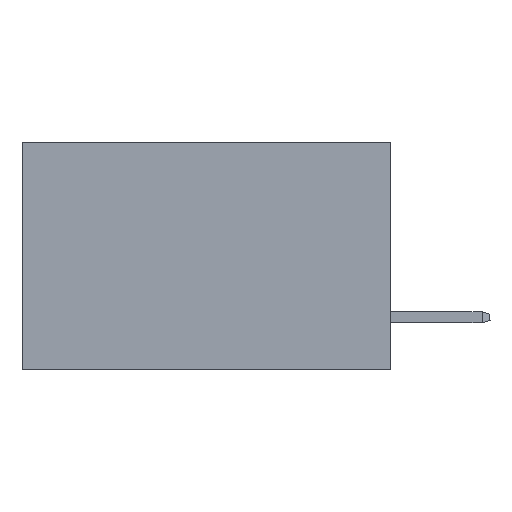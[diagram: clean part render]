
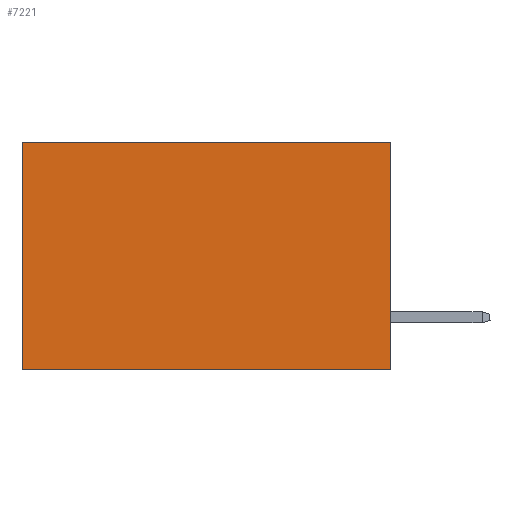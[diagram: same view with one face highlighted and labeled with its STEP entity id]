
A CAD part, left-side view. The second image highlights one B-rep face of the part: STEP entity #7221.
In plain terms, the highlighted planar face has unit normal (-1, 0, 0).
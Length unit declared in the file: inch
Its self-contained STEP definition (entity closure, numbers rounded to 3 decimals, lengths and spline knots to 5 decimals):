
#530 = CARTESIAN_POINT ( 'NONE',  ( 0.2875, 0.6, 0. ) ) ;
#2797 = DIRECTION ( 'NONE',  ( 0., 0., -1. ) ) ;
#3130 = LINE ( 'NONE', #530, #23320 ) ;
#3460 = VERTEX_POINT ( 'NONE', #29078 ) ;
#5425 = VERTEX_POINT ( 'NONE', #13934 ) ;
#5978 = FACE_OUTER_BOUND ( 'NONE', #24922, .T. ) ;
#6618 = CARTESIAN_POINT ( 'NONE',  ( 0.2875, 0.6, 0. ) ) ;
#7221 = ADVANCED_FACE ( 'NONE', ( #5978 ), #30137, .F. ) ;
#7274 = EDGE_CURVE ( 'NONE', #8985, #5425, #12591, .T. ) ;
#7565 = VECTOR ( 'NONE', #7709, 39.37008 ) ;
#7598 = CARTESIAN_POINT ( 'NONE',  ( 0.2875, 0., 0. ) ) ;
#7621 = DIRECTION ( 'NONE',  ( 1., 0., 0. ) ) ;
#7709 = DIRECTION ( 'NONE',  ( 0., 1., 0. ) ) ;
#8985 = VERTEX_POINT ( 'NONE', #9465 ) ;
#9465 = CARTESIAN_POINT ( 'NONE',  ( 0.2875, 0., -0.37 ) ) ;
#10188 = CARTESIAN_POINT ( 'NONE',  ( 0.2875, 0., -0.37 ) ) ;
#10444 = VECTOR ( 'NONE', #11408, 39.37008 ) ;
#11408 = DIRECTION ( 'NONE',  ( 0., 0., -1. ) ) ;
#12512 = ORIENTED_EDGE ( 'NONE', *, *, #13405, .T. ) ;
#12591 = LINE ( 'NONE', #10188, #16375 ) ;
#13405 = EDGE_CURVE ( 'NONE', #20441, #5425, #3130, .T. ) ;
#13934 = CARTESIAN_POINT ( 'NONE',  ( 0.2875, 0.6, -0.37 ) ) ;
#13938 = EDGE_CURVE ( 'NONE', #3460, #20441, #26909, .T. ) ;
#14332 = AXIS2_PLACEMENT_3D ( 'NONE', #7598, #7621, #20431 ) ;
#15005 = EDGE_CURVE ( 'NONE', #3460, #8985, #15693, .T. ) ;
#15356 = ORIENTED_EDGE ( 'NONE', *, *, #13938, .T. ) ;
#15693 = LINE ( 'NONE', #30010, #10444 ) ;
#16375 = VECTOR ( 'NONE', #24616, 39.37008 ) ;
#16640 = ORIENTED_EDGE ( 'NONE', *, *, #15005, .F. ) ;
#17192 = CARTESIAN_POINT ( 'NONE',  ( 0.2875, 0., 0. ) ) ;
#20431 = DIRECTION ( 'NONE',  ( 0., 0., -1. ) ) ;
#20441 = VERTEX_POINT ( 'NONE', #6618 ) ;
#23320 = VECTOR ( 'NONE', #2797, 39.37008 ) ;
#24616 = DIRECTION ( 'NONE',  ( 0., 1., 0. ) ) ;
#24922 = EDGE_LOOP ( 'NONE', ( #12512, #26808, #16640, #15356 ) ) ;
#26808 = ORIENTED_EDGE ( 'NONE', *, *, #7274, .F. ) ;
#26909 = LINE ( 'NONE', #17192, #7565 ) ;
#29078 = CARTESIAN_POINT ( 'NONE',  ( 0.2875, 0., 0. ) ) ;
#30010 = CARTESIAN_POINT ( 'NONE',  ( 0.2875, 0., 0. ) ) ;
#30137 = PLANE ( 'NONE',  #14332 ) ;
